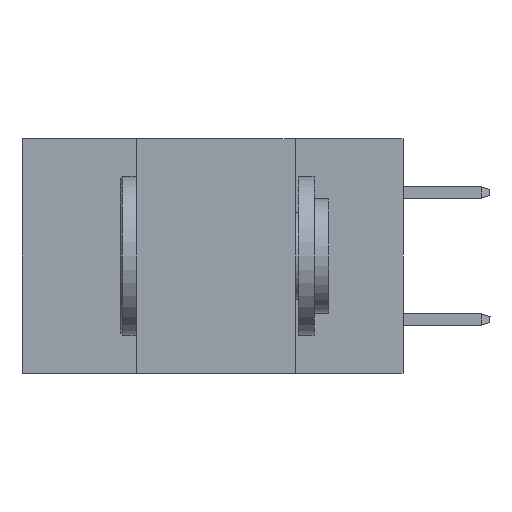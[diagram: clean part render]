
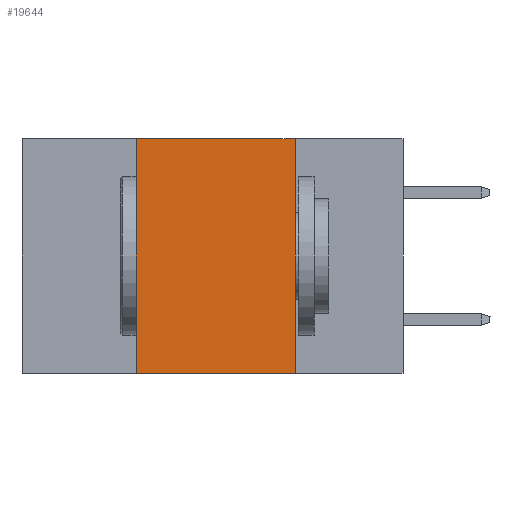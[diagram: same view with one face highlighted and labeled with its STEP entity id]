
A CAD part, left-side view. The second image highlights one B-rep face of the part: STEP entity #19644.
In plain terms, the highlighted planar face has unit normal (-1, 0, 0).
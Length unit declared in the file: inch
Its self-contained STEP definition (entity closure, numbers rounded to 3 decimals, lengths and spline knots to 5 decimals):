
#869 = EDGE_CURVE ( 'NONE', #13209, #20785, #28787, .T. ) ;
#1615 = DIRECTION ( 'NONE',  ( 0., 0., 1. ) ) ;
#1632 = AXIS2_PLACEMENT_3D ( 'NONE', #23008, #29835, #15724 ) ;
#2018 = CARTESIAN_POINT ( 'NONE',  ( 0., 0.42, 0. ) ) ;
#2123 = LINE ( 'NONE', #11577, #15298 ) ;
#6211 = CARTESIAN_POINT ( 'NONE',  ( 0., 0.42, 0. ) ) ;
#7611 = EDGE_CURVE ( 'NONE', #13209, #10654, #29510, .T. ) ;
#9882 = DIRECTION ( 'NONE',  ( 0., -1., 0. ) ) ;
#9991 = CARTESIAN_POINT ( 'NONE',  ( 0., 0.6, -0.37 ) ) ;
#10547 = LINE ( 'NONE', #20026, #14179 ) ;
#10654 = VERTEX_POINT ( 'NONE', #2018 ) ;
#11577 = CARTESIAN_POINT ( 'NONE',  ( 0., 0.17, 0. ) ) ;
#12521 = CARTESIAN_POINT ( 'NONE',  ( 0., 0.17, 0. ) ) ;
#13209 = VERTEX_POINT ( 'NONE', #18313 ) ;
#13538 = FACE_OUTER_BOUND ( 'NONE', #27940, .T. ) ;
#14088 = CARTESIAN_POINT ( 'NONE',  ( 0., 0.17, -0.37 ) ) ;
#14179 = VECTOR ( 'NONE', #9882, 39.37008 ) ;
#14830 = DIRECTION ( 'NONE',  ( 0., -1., 0. ) ) ;
#14906 = ORIENTED_EDGE ( 'NONE', *, *, #30375, .F. ) ;
#15298 = VECTOR ( 'NONE', #16373, 39.37008 ) ;
#15724 = DIRECTION ( 'NONE',  ( 0., 0., -1. ) ) ;
#15770 = EDGE_CURVE ( 'NONE', #25896, #20785, #2123, .T. ) ;
#16373 = DIRECTION ( 'NONE',  ( 0., 0., -1. ) ) ;
#18313 = CARTESIAN_POINT ( 'NONE',  ( 0., 0.42, -0.37 ) ) ;
#19390 = VECTOR ( 'NONE', #14830, 39.37008 ) ;
#19644 = ADVANCED_FACE ( 'NONE', ( #13538 ), #29530, .F. ) ;
#19679 = VECTOR ( 'NONE', #1615, 39.37008 ) ;
#20026 = CARTESIAN_POINT ( 'NONE',  ( 0., 0.6, 0. ) ) ;
#20707 = ORIENTED_EDGE ( 'NONE', *, *, #869, .T. ) ;
#20785 = VERTEX_POINT ( 'NONE', #14088 ) ;
#23008 = CARTESIAN_POINT ( 'NONE',  ( 0., 0.6, 0. ) ) ;
#24704 = ORIENTED_EDGE ( 'NONE', *, *, #7611, .F. ) ;
#25896 = VERTEX_POINT ( 'NONE', #12521 ) ;
#27717 = ORIENTED_EDGE ( 'NONE', *, *, #15770, .F. ) ;
#27940 = EDGE_LOOP ( 'NONE', ( #27717, #14906, #24704, #20707 ) ) ;
#28787 = LINE ( 'NONE', #9991, #19390 ) ;
#29510 = LINE ( 'NONE', #6211, #19679 ) ;
#29530 = PLANE ( 'NONE',  #1632 ) ;
#29835 = DIRECTION ( 'NONE',  ( 1., 0., 0. ) ) ;
#30375 = EDGE_CURVE ( 'NONE', #10654, #25896, #10547, .T. ) ;
